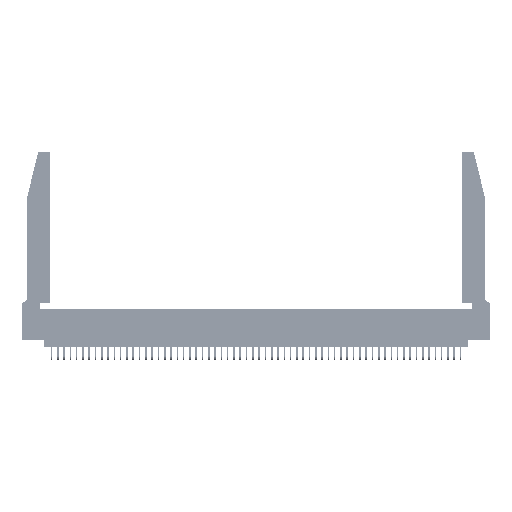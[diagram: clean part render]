
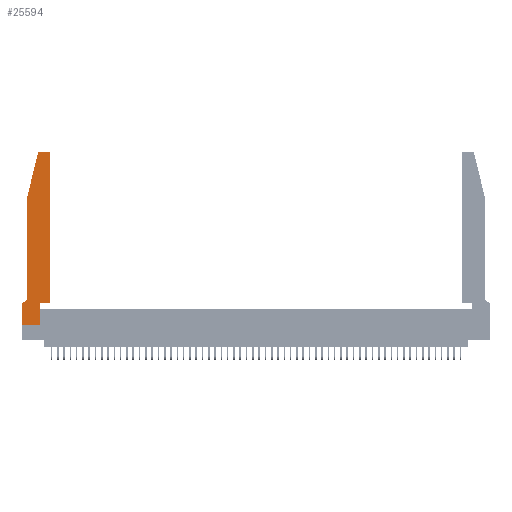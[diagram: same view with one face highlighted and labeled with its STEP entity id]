
A CAD part, top view. The second image highlights one B-rep face of the part: STEP entity #25594.
In plain terms, the highlighted planar face has unit normal (0, 0, 1).
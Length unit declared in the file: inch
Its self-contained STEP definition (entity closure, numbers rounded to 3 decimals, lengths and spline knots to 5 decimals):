
#13 = ORIENTED_EDGE ( 'NONE', *, *, #27381, .T. ) ;
#408 = VECTOR ( 'NONE', #7231, 39.37008 ) ;
#915 = LINE ( 'NONE', #10335, #3622 ) ;
#2465 = VECTOR ( 'NONE', #29936, 39.37008 ) ;
#2705 = CARTESIAN_POINT ( 'NONE',  ( 0.2865, 0., 0.37 ) ) ;
#2845 = CARTESIAN_POINT ( 'NONE',  ( 0.0755, 2., 0.37 ) ) ;
#2949 = CARTESIAN_POINT ( 'NONE',  ( 0.2605, 2.75, 0.37 ) ) ;
#3622 = VECTOR ( 'NONE', #40201, 39.37008 ) ;
#4319 = CARTESIAN_POINT ( 'NONE',  ( 0., 0., 0.37 ) ) ;
#4371 = CARTESIAN_POINT ( 'NONE',  ( 0.25487, 2.72718, 0.37 ) ) ;
#4634 = DIRECTION ( 'NONE',  ( -1., 0., 0. ) ) ;
#4652 = VERTEX_POINT ( 'NONE', #36758 ) ;
#4897 = CARTESIAN_POINT ( 'NONE',  ( 0.284, 2.75, 0.37 ) ) ;
#4930 = EDGE_CURVE ( 'NONE', #52737, #4652, #46494, .T. ) ;
#5006 = VECTOR ( 'NONE', #50738, 39.37008 ) ;
#5229 = VERTEX_POINT ( 'NONE', #32053 ) ;
#5261 = ORIENTED_EDGE ( 'NONE', *, *, #4930, .T. ) ;
#5569 = VERTEX_POINT ( 'NONE', #4371 ) ;
#5821 = CARTESIAN_POINT ( 'NONE',  ( 0.4505, 0.35, 0.37 ) ) ;
#6837 = VERTEX_POINT ( 'NONE', #34367 ) ;
#7015 = CARTESIAN_POINT ( 'NONE',  ( 0.4205, 2.72, 0.37 ) ) ;
#7231 = DIRECTION ( 'NONE',  ( -1., 0., 0. ) ) ;
#7846 = EDGE_CURVE ( 'NONE', #5229, #11514, #47108, .T. ) ;
#9087 = EDGE_CURVE ( 'NONE', #32122, #30789, #915, .T. ) ;
#9428 = ORIENTED_EDGE ( 'NONE', *, *, #13910, .T. ) ;
#10335 = CARTESIAN_POINT ( 'NONE',  ( 0.2865, 0.35, 0.37 ) ) ;
#10649 = ORIENTED_EDGE ( 'NONE', *, *, #31372, .T. ) ;
#11143 = VECTOR ( 'NONE', #35695, 39.37008 ) ;
#11317 = DIRECTION ( 'NONE',  ( 1., 0., 0. ) ) ;
#11514 = VERTEX_POINT ( 'NONE', #4897 ) ;
#11873 = AXIS2_PLACEMENT_3D ( 'NONE', #39258, #13677, #43504 ) ;
#12345 = VERTEX_POINT ( 'NONE', #45695 ) ;
#13418 = ORIENTED_EDGE ( 'NONE', *, *, #19990, .T. ) ;
#13448 = AXIS2_PLACEMENT_3D ( 'NONE', #7015, #36898, #11317 ) ;
#13677 = DIRECTION ( 'NONE',  ( 0., 0., 1. ) ) ;
#13910 = EDGE_CURVE ( 'NONE', #11514, #5569, #36422, .T. ) ;
#14174 = VECTOR ( 'NONE', #49310, 39.37008 ) ;
#15430 = ORIENTED_EDGE ( 'NONE', *, *, #31657, .T. ) ;
#15998 = CARTESIAN_POINT ( 'NONE',  ( 0.0755, 0.42, 0.37 ) ) ;
#16251 = DIRECTION ( 'NONE',  ( 0., 0., -1. ) ) ;
#17898 = AXIS2_PLACEMENT_3D ( 'NONE', #41794, #16251, #46051 ) ;
#19604 = AXIS2_PLACEMENT_3D ( 'NONE', #38584, #47106, #21646 ) ;
#19828 = CARTESIAN_POINT ( 'NONE',  ( 0.2865, 0.35, 0.37 ) ) ;
#19990 = EDGE_CURVE ( 'NONE', #4652, #6837, #33857, .T. ) ;
#20744 = CIRCLE ( 'NONE', #13448, 0.03 ) ;
#21188 = LINE ( 'NONE', #5821, #11143 ) ;
#21444 = LINE ( 'NONE', #2845, #31472 ) ;
#21646 = DIRECTION ( 'NONE',  ( 1., 0., 0. ) ) ;
#22473 = EDGE_CURVE ( 'NONE', #6837, #32122, #48165, .T. ) ;
#23483 = ORIENTED_EDGE ( 'NONE', *, *, #22473, .T. ) ;
#25228 = VECTOR ( 'NONE', #4634, 39.37008 ) ;
#25594 = ADVANCED_FACE ( 'NONE', ( #45258 ), #34311, .T. ) ;
#27102 = VECTOR ( 'NONE', #36364, 39.37008 ) ;
#27381 = EDGE_CURVE ( 'NONE', #31527, #52737, #38488, .T. ) ;
#27768 = LINE ( 'NONE', #46530, #5006 ) ;
#28005 = CARTESIAN_POINT ( 'NONE',  ( 0., 0., 0.37 ) ) ;
#28446 = DIRECTION ( 'NONE',  ( -0.239, -0.971, 0. ) ) ;
#28936 = CARTESIAN_POINT ( 'NONE',  ( 0.4505, 0.35, 0.37 ) ) ;
#29936 = DIRECTION ( 'NONE',  ( 0., -1., 0. ) ) ;
#30225 = CARTESIAN_POINT ( 'NONE',  ( 0.0755, 0.35, 0.37 ) ) ;
#30594 = CARTESIAN_POINT ( 'NONE',  ( 0.0055, 0.35, 0.37 ) ) ;
#30789 = VERTEX_POINT ( 'NONE', #19828 ) ;
#31372 = EDGE_CURVE ( 'NONE', #30789, #43292, #38399, .T. ) ;
#31472 = VECTOR ( 'NONE', #28446, 39.37008 ) ;
#31527 = VERTEX_POINT ( 'NONE', #15998 ) ;
#31657 = EDGE_CURVE ( 'NONE', #35126, #31527, #27768, .T. ) ;
#31917 = CARTESIAN_POINT ( 'NONE',  ( 0.4505, 0.35, 0.37 ) ) ;
#32053 = CARTESIAN_POINT ( 'NONE',  ( 0.4205, 2.75, 0.37 ) ) ;
#32122 = VERTEX_POINT ( 'NONE', #2705 ) ;
#33777 = ORIENTED_EDGE ( 'NONE', *, *, #53416, .T. ) ;
#33857 = LINE ( 'NONE', #4319, #2465 ) ;
#34311 = PLANE ( 'NONE',  #19604 ) ;
#34367 = CARTESIAN_POINT ( 'NONE',  ( 0., 0., 0.37 ) ) ;
#34537 = ORIENTED_EDGE ( 'NONE', *, *, #9087, .T. ) ;
#35126 = VERTEX_POINT ( 'NONE', #40259 ) ;
#35184 = EDGE_CURVE ( 'NONE', #12345, #5229, #20744, .T. ) ;
#35695 = DIRECTION ( 'NONE',  ( 0., 1., 0. ) ) ;
#36364 = DIRECTION ( 'NONE',  ( 1., 0., 0. ) ) ;
#36422 = CIRCLE ( 'NONE', #11873, 0.03 ) ;
#36758 = CARTESIAN_POINT ( 'NONE',  ( 0., 0.35, 0.37 ) ) ;
#36898 = DIRECTION ( 'NONE',  ( 0., 0., 1. ) ) ;
#38399 = LINE ( 'NONE', #31917, #27102 ) ;
#38488 = CIRCLE ( 'NONE', #17898, 0.07 ) ;
#38584 = CARTESIAN_POINT ( 'NONE',  ( 0., 0.35, 0.37 ) ) ;
#39258 = CARTESIAN_POINT ( 'NONE',  ( 0.284, 2.72, 0.37 ) ) ;
#40201 = DIRECTION ( 'NONE',  ( 0., 1., 0. ) ) ;
#40259 = CARTESIAN_POINT ( 'NONE',  ( 0.0755, 2., 0.37 ) ) ;
#41794 = CARTESIAN_POINT ( 'NONE',  ( 0.0055, 0.42, 0.37 ) ) ;
#42439 = ORIENTED_EDGE ( 'NONE', *, *, #35184, .T. ) ;
#43292 = VERTEX_POINT ( 'NONE', #28936 ) ;
#43504 = DIRECTION ( 'NONE',  ( 1., 0., 0. ) ) ;
#44773 = ORIENTED_EDGE ( 'NONE', *, *, #7846, .T. ) ;
#45258 = FACE_OUTER_BOUND ( 'NONE', #47502, .T. ) ;
#45695 = CARTESIAN_POINT ( 'NONE',  ( 0.4505, 2.72, 0.37 ) ) ;
#46051 = DIRECTION ( 'NONE',  ( -1., 0., 0. ) ) ;
#46494 = LINE ( 'NONE', #30225, #25228 ) ;
#46530 = CARTESIAN_POINT ( 'NONE',  ( 0.0755, 2., 0.37 ) ) ;
#47106 = DIRECTION ( 'NONE',  ( 0., 0., 1. ) ) ;
#47108 = LINE ( 'NONE', #2949, #408 ) ;
#47502 = EDGE_LOOP ( 'NONE', ( #44773, #9428, #49395, #15430, #13, #5261, #13418, #23483, #34537, #10649, #33777, #42439 ) ) ;
#48165 = LINE ( 'NONE', #28005, #14174 ) ;
#49310 = DIRECTION ( 'NONE',  ( 1., 0., 0. ) ) ;
#49395 = ORIENTED_EDGE ( 'NONE', *, *, #50458, .T. ) ;
#50458 = EDGE_CURVE ( 'NONE', #5569, #35126, #21444, .T. ) ;
#50738 = DIRECTION ( 'NONE',  ( 0., -1., 0. ) ) ;
#52737 = VERTEX_POINT ( 'NONE', #30594 ) ;
#53416 = EDGE_CURVE ( 'NONE', #43292, #12345, #21188, .T. ) ;
